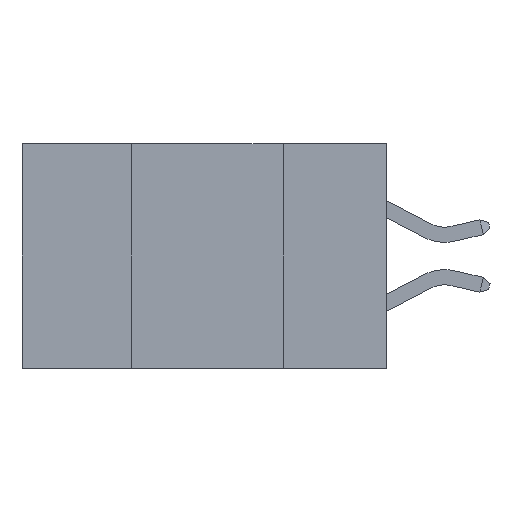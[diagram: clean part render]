
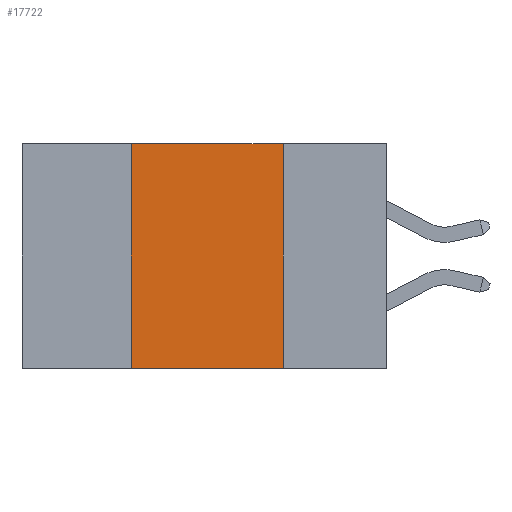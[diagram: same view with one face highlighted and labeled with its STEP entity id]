
A CAD part, left-side view. The second image highlights one B-rep face of the part: STEP entity #17722.
In plain terms, the highlighted planar face has unit normal (-1, 0, 0).
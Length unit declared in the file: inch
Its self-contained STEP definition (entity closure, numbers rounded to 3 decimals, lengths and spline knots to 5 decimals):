
#373 = EDGE_CURVE ( 'NONE', #13436, #10518, #19085, .T. ) ;
#550 = VERTEX_POINT ( 'NONE', #5038 ) ;
#1502 = ORIENTED_EDGE ( 'NONE', *, *, #373, .F. ) ;
#2816 = DIRECTION ( 'NONE',  ( 0., 0., 1. ) ) ;
#3250 = LINE ( 'NONE', #19610, #16041 ) ;
#3801 = LINE ( 'NONE', #15503, #7918 ) ;
#4922 = ORIENTED_EDGE ( 'NONE', *, *, #17500, .F. ) ;
#5038 = CARTESIAN_POINT ( 'NONE',  ( 0., 0.42, -0.37 ) ) ;
#5388 = CARTESIAN_POINT ( 'NONE',  ( 0., 0.17, -0.37 ) ) ;
#5844 = ORIENTED_EDGE ( 'NONE', *, *, #8659, .F. ) ;
#6233 = DIRECTION ( 'NONE',  ( 0., 0., -1. ) ) ;
#6388 = DIRECTION ( 'NONE',  ( 0., -1., 0. ) ) ;
#6742 = CARTESIAN_POINT ( 'NONE',  ( 0., 0.17, 0. ) ) ;
#7210 = AXIS2_PLACEMENT_3D ( 'NONE', #16505, #18619, #6233 ) ;
#7918 = VECTOR ( 'NONE', #10796, 39.37008 ) ;
#8487 = VECTOR ( 'NONE', #6388, 39.37008 ) ;
#8659 = EDGE_CURVE ( 'NONE', #12065, #13436, #12343, .T. ) ;
#10518 = VERTEX_POINT ( 'NONE', #5388 ) ;
#10559 = EDGE_LOOP ( 'NONE', ( #1502, #5844, #4922, #17306 ) ) ;
#10796 = DIRECTION ( 'NONE',  ( 0., -1., 0. ) ) ;
#11057 = EDGE_CURVE ( 'NONE', #550, #10518, #3801, .T. ) ;
#12060 = VECTOR ( 'NONE', #19202, 39.37008 ) ;
#12065 = VERTEX_POINT ( 'NONE', #17318 ) ;
#12343 = LINE ( 'NONE', #18848, #8487 ) ;
#13436 = VERTEX_POINT ( 'NONE', #14419 ) ;
#14419 = CARTESIAN_POINT ( 'NONE',  ( 0., 0.17, 0. ) ) ;
#15419 = PLANE ( 'NONE',  #7210 ) ;
#15503 = CARTESIAN_POINT ( 'NONE',  ( 0., 0.6, -0.37 ) ) ;
#16041 = VECTOR ( 'NONE', #2816, 39.37008 ) ;
#16505 = CARTESIAN_POINT ( 'NONE',  ( 0., 0.6, 0. ) ) ;
#17306 = ORIENTED_EDGE ( 'NONE', *, *, #11057, .T. ) ;
#17318 = CARTESIAN_POINT ( 'NONE',  ( 0., 0.42, 0. ) ) ;
#17500 = EDGE_CURVE ( 'NONE', #550, #12065, #3250, .T. ) ;
#17722 = ADVANCED_FACE ( 'NONE', ( #18052 ), #15419, .F. ) ;
#18052 = FACE_OUTER_BOUND ( 'NONE', #10559, .T. ) ;
#18619 = DIRECTION ( 'NONE',  ( 1., 0., 0. ) ) ;
#18848 = CARTESIAN_POINT ( 'NONE',  ( 0., 0.6, 0. ) ) ;
#19085 = LINE ( 'NONE', #6742, #12060 ) ;
#19202 = DIRECTION ( 'NONE',  ( 0., 0., -1. ) ) ;
#19610 = CARTESIAN_POINT ( 'NONE',  ( 0., 0.42, 0. ) ) ;
